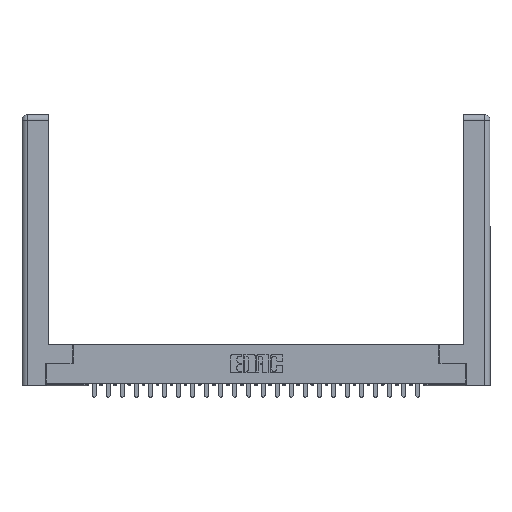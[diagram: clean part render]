
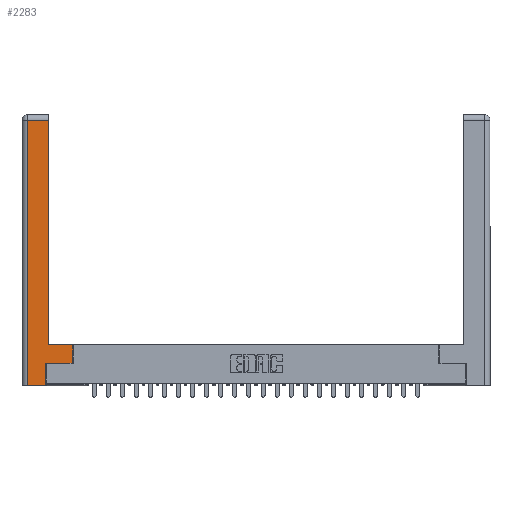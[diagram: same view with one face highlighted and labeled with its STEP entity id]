
A CAD part, top view. The second image highlights one B-rep face of the part: STEP entity #2283.
In plain terms, the highlighted planar face has unit normal (0, 0, 1).
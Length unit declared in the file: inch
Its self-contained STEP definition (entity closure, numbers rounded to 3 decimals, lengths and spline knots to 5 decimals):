
#367 = VERTEX_POINT ( 'NONE', #14580 ) ;
#687 = CARTESIAN_POINT ( 'NONE',  ( 0.295, 2.94, 0. ) ) ;
#859 = DIRECTION ( 'NONE',  ( 1., 0., 0. ) ) ;
#1672 = LINE ( 'NONE', #8984, #3508 ) ;
#1993 = VECTOR ( 'NONE', #6541, 39.37008 ) ;
#2283 = ADVANCED_FACE ( 'NONE', ( #27769 ), #7082, .F. ) ;
#2949 = DIRECTION ( 'NONE',  ( 0., 1., 0. ) ) ;
#3508 = VECTOR ( 'NONE', #7608, 39.37008 ) ;
#4102 = CARTESIAN_POINT ( 'NONE',  ( 0.565, 0.245, 0. ) ) ;
#6291 = CARTESIAN_POINT ( 'NONE',  ( 0.565, 0.245, 0. ) ) ;
#6541 = DIRECTION ( 'NONE',  ( 0., 1., 0. ) ) ;
#6548 = LINE ( 'NONE', #20922, #26535 ) ;
#6600 = EDGE_CURVE ( 'NONE', #18662, #7726, #7129, .T. ) ;
#7082 = PLANE ( 'NONE',  #20449 ) ;
#7129 = LINE ( 'NONE', #6291, #9716 ) ;
#7608 = DIRECTION ( 'NONE',  ( -1., 0., 0. ) ) ;
#7726 = VERTEX_POINT ( 'NONE', #4102 ) ;
#8404 = LINE ( 'NONE', #24211, #24703 ) ;
#8467 = DIRECTION ( 'NONE',  ( 0., -1., 0. ) ) ;
#8984 = CARTESIAN_POINT ( 'NONE',  ( 0.0615, 2.94, 0. ) ) ;
#9154 = DIRECTION ( 'NONE',  ( -1., 0., 0. ) ) ;
#9358 = DIRECTION ( 'NONE',  ( 0., 0., -1. ) ) ;
#9716 = VECTOR ( 'NONE', #27813, 39.37008 ) ;
#10010 = CARTESIAN_POINT ( 'NONE',  ( 0.295, 3., 0. ) ) ;
#10111 = ORIENTED_EDGE ( 'NONE', *, *, #24347, .T. ) ;
#10178 = VERTEX_POINT ( 'NONE', #14297 ) ;
#10532 = LINE ( 'NONE', #24309, #13885 ) ;
#10550 = CARTESIAN_POINT ( 'NONE',  ( 0.0615, 0., 0. ) ) ;
#10586 = CARTESIAN_POINT ( 'NONE',  ( 0.565, 0.45, 0. ) ) ;
#12260 = VERTEX_POINT ( 'NONE', #18156 ) ;
#12333 = ORIENTED_EDGE ( 'NONE', *, *, #27780, .T. ) ;
#12555 = ORIENTED_EDGE ( 'NONE', *, *, #13194, .T. ) ;
#12980 = ORIENTED_EDGE ( 'NONE', *, *, #28894, .T. ) ;
#13194 = EDGE_CURVE ( 'NONE', #12260, #26720, #10532, .T. ) ;
#13831 = ORIENTED_EDGE ( 'NONE', *, *, #19324, .T. ) ;
#13885 = VECTOR ( 'NONE', #859, 39.37008 ) ;
#14297 = CARTESIAN_POINT ( 'NONE',  ( 0.295, 0.45, 0. ) ) ;
#14580 = CARTESIAN_POINT ( 'NONE',  ( 0.565, 0.45, 0. ) ) ;
#14888 = VERTEX_POINT ( 'NONE', #687 ) ;
#16083 = EDGE_CURVE ( 'NONE', #26720, #18662, #8404, .T. ) ;
#16265 = EDGE_LOOP ( 'NONE', ( #12333, #12980, #20739, #12555, #30308, #17505, #13831, #10111 ) ) ;
#16497 = CARTESIAN_POINT ( 'NONE',  ( 0., 0., 0. ) ) ;
#17505 = ORIENTED_EDGE ( 'NONE', *, *, #6600, .T. ) ;
#18004 = VECTOR ( 'NONE', #26467, 39.37008 ) ;
#18156 = CARTESIAN_POINT ( 'NONE',  ( 0.0615, 0., 0. ) ) ;
#18662 = VERTEX_POINT ( 'NONE', #22021 ) ;
#19324 = EDGE_CURVE ( 'NONE', #7726, #367, #23395, .T. ) ;
#19665 = VECTOR ( 'NONE', #8467, 39.37008 ) ;
#19851 = EDGE_CURVE ( 'NONE', #28081, #12260, #24491, .T. ) ;
#20449 = AXIS2_PLACEMENT_3D ( 'NONE', #16497, #9358, #9154 ) ;
#20739 = ORIENTED_EDGE ( 'NONE', *, *, #19851, .T. ) ;
#20922 = CARTESIAN_POINT ( 'NONE',  ( 0.295, 0.45, 0. ) ) ;
#21691 = CARTESIAN_POINT ( 'NONE',  ( 0.265, 0., 0. ) ) ;
#22021 = CARTESIAN_POINT ( 'NONE',  ( 0.265, 0.245, 0. ) ) ;
#23276 = DIRECTION ( 'NONE',  ( -1., 0., 0. ) ) ;
#23395 = LINE ( 'NONE', #10586, #1993 ) ;
#23898 = LINE ( 'NONE', #10010, #18004 ) ;
#24211 = CARTESIAN_POINT ( 'NONE',  ( 0.265, 0.245, 0. ) ) ;
#24309 = CARTESIAN_POINT ( 'NONE',  ( 0.265, 0., 0. ) ) ;
#24347 = EDGE_CURVE ( 'NONE', #367, #10178, #6548, .T. ) ;
#24491 = LINE ( 'NONE', #10550, #19665 ) ;
#24703 = VECTOR ( 'NONE', #2949, 39.37008 ) ;
#26467 = DIRECTION ( 'NONE',  ( 0., 1., 0. ) ) ;
#26535 = VECTOR ( 'NONE', #23276, 39.37008 ) ;
#26720 = VERTEX_POINT ( 'NONE', #21691 ) ;
#27769 = FACE_OUTER_BOUND ( 'NONE', #16265, .T. ) ;
#27780 = EDGE_CURVE ( 'NONE', #10178, #14888, #23898, .T. ) ;
#27813 = DIRECTION ( 'NONE',  ( 1., 0., 0. ) ) ;
#28081 = VERTEX_POINT ( 'NONE', #28771 ) ;
#28771 = CARTESIAN_POINT ( 'NONE',  ( 0.0615, 2.94, 0. ) ) ;
#28894 = EDGE_CURVE ( 'NONE', #14888, #28081, #1672, .T. ) ;
#30308 = ORIENTED_EDGE ( 'NONE', *, *, #16083, .T. ) ;
